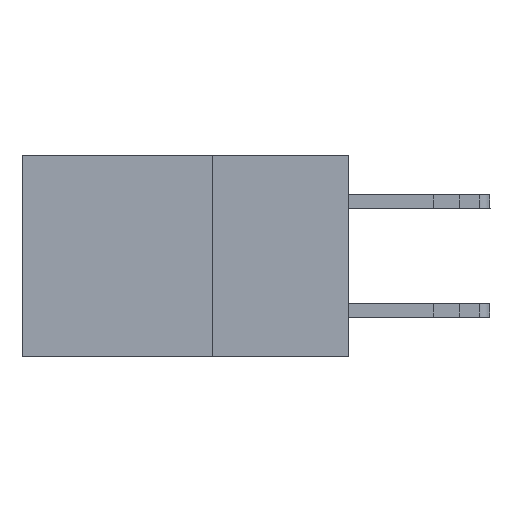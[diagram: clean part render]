
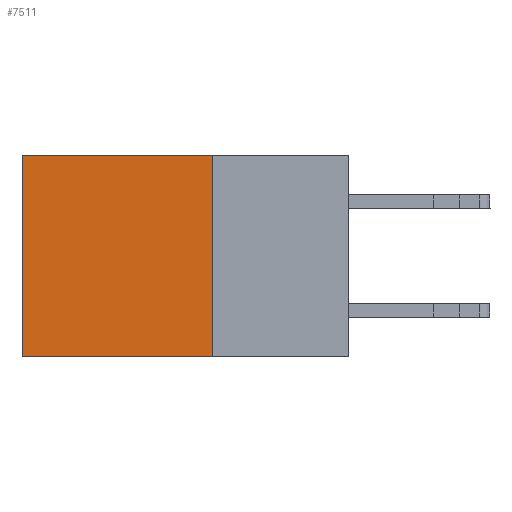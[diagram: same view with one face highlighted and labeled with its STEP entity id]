
A CAD part, left-side view. The second image highlights one B-rep face of the part: STEP entity #7511.
In plain terms, the highlighted planar face has unit normal (-1, 0, 0).
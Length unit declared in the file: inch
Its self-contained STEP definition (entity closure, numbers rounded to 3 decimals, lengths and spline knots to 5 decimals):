
#163 = DIRECTION ( 'NONE',  ( 0., 1., 0. ) ) ;
#1760 = EDGE_CURVE ( 'NONE', #12713, #6635, #4288, .T. ) ;
#1825 = CARTESIAN_POINT ( 'NONE',  ( 0.2615, 0.25, -0.37 ) ) ;
#2058 = ORIENTED_EDGE ( 'NONE', *, *, #1760, .T. ) ;
#2636 = ORIENTED_EDGE ( 'NONE', *, *, #3324, .T. ) ;
#2646 = CARTESIAN_POINT ( 'NONE',  ( 0.2615, 0.25, -0.37 ) ) ;
#2959 = CARTESIAN_POINT ( 'NONE',  ( 0.2615, 0.6, -0.37 ) ) ;
#3324 = EDGE_CURVE ( 'NONE', #17166, #12713, #18132, .T. ) ;
#3657 = AXIS2_PLACEMENT_3D ( 'NONE', #14464, #11388, #10275 ) ;
#4288 = LINE ( 'NONE', #2959, #15048 ) ;
#6084 = FACE_OUTER_BOUND ( 'NONE', #6837, .T. ) ;
#6635 = VERTEX_POINT ( 'NONE', #17290 ) ;
#6763 = DIRECTION ( 'NONE',  ( 0., 0., -1. ) ) ;
#6837 = EDGE_LOOP ( 'NONE', ( #2058, #9792, #12041, #2636 ) ) ;
#7511 = ADVANCED_FACE ( 'NONE', ( #6084 ), #11657, .F. ) ;
#7772 = VECTOR ( 'NONE', #15162, 39.37008 ) ;
#9792 = ORIENTED_EDGE ( 'NONE', *, *, #12799, .F. ) ;
#10275 = DIRECTION ( 'NONE',  ( 0., 0., -1. ) ) ;
#10847 = LINE ( 'NONE', #2646, #11638 ) ;
#11156 = CARTESIAN_POINT ( 'NONE',  ( 0.2615, 0.25, 0. ) ) ;
#11388 = DIRECTION ( 'NONE',  ( 1., 0., 0. ) ) ;
#11638 = VECTOR ( 'NONE', #6763, 39.37008 ) ;
#11657 = PLANE ( 'NONE',  #3657 ) ;
#12041 = ORIENTED_EDGE ( 'NONE', *, *, #16197, .F. ) ;
#12713 = VERTEX_POINT ( 'NONE', #13971 ) ;
#12799 = EDGE_CURVE ( 'NONE', #18347, #6635, #13301, .T. ) ;
#12968 = VECTOR ( 'NONE', #163, 39.37008 ) ;
#13301 = LINE ( 'NONE', #1825, #12968 ) ;
#13971 = CARTESIAN_POINT ( 'NONE',  ( 0.2615, 0.6, 0. ) ) ;
#14464 = CARTESIAN_POINT ( 'NONE',  ( 0.2615, 0.25, -0.37 ) ) ;
#15048 = VECTOR ( 'NONE', #15808, 39.37008 ) ;
#15162 = DIRECTION ( 'NONE',  ( 0., 1., 0. ) ) ;
#15373 = CARTESIAN_POINT ( 'NONE',  ( 0.2615, 0.25, -0.37 ) ) ;
#15808 = DIRECTION ( 'NONE',  ( 0., 0., -1. ) ) ;
#16197 = EDGE_CURVE ( 'NONE', #17166, #18347, #10847, .T. ) ;
#16296 = CARTESIAN_POINT ( 'NONE',  ( 0.2615, 0.25, 0. ) ) ;
#17166 = VERTEX_POINT ( 'NONE', #16296 ) ;
#17290 = CARTESIAN_POINT ( 'NONE',  ( 0.2615, 0.6, -0.37 ) ) ;
#18132 = LINE ( 'NONE', #11156, #7772 ) ;
#18347 = VERTEX_POINT ( 'NONE', #15373 ) ;
